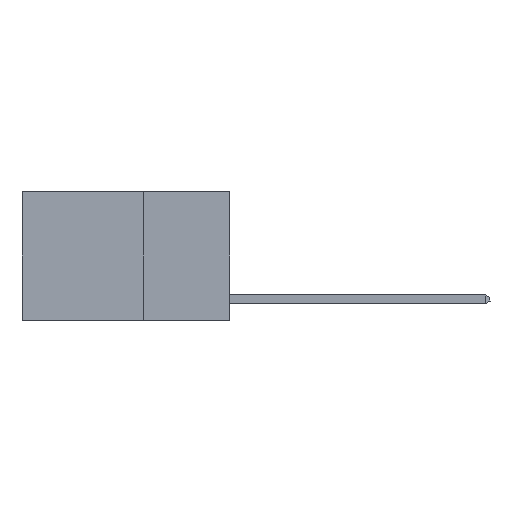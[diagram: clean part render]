
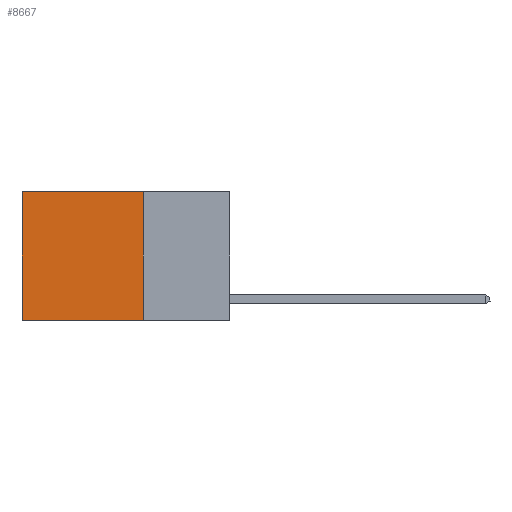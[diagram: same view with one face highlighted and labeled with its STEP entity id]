
A CAD part, left-side view. The second image highlights one B-rep face of the part: STEP entity #8667.
In plain terms, the highlighted planar face has unit normal (-1, 0, 0).
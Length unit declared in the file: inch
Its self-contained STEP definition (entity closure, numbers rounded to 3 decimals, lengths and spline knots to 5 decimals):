
#802 = VECTOR ( 'NONE', #3704, 39.37008 ) ;
#1063 = VECTOR ( 'NONE', #5669, 39.37008 ) ;
#1593 = AXIS2_PLACEMENT_3D ( 'NONE', #11629, #4308, #6087 ) ;
#1999 = VECTOR ( 'NONE', #6396, 39.37008 ) ;
#2716 = VERTEX_POINT ( 'NONE', #7676 ) ;
#2733 = CARTESIAN_POINT ( 'NONE',  ( 0.2625, 0.25, 0. ) ) ;
#3064 = EDGE_CURVE ( 'NONE', #2716, #7961, #5777, .T. ) ;
#3219 = LINE ( 'NONE', #4077, #10288 ) ;
#3458 = PLANE ( 'NONE',  #1593 ) ;
#3704 = DIRECTION ( 'NONE',  ( 0., 0., -1. ) ) ;
#4077 = CARTESIAN_POINT ( 'NONE',  ( 0.2625, 0.25, -0.37 ) ) ;
#4201 = ORIENTED_EDGE ( 'NONE', *, *, #3064, .T. ) ;
#4308 = DIRECTION ( 'NONE',  ( 1., 0., 0. ) ) ;
#4345 = LINE ( 'NONE', #11721, #1999 ) ;
#4838 = DIRECTION ( 'NONE',  ( 0., 1., 0. ) ) ;
#5084 = ORIENTED_EDGE ( 'NONE', *, *, #11746, .T. ) ;
#5361 = EDGE_LOOP ( 'NONE', ( #5084, #11357, #8856, #4201 ) ) ;
#5669 = DIRECTION ( 'NONE',  ( 0., 1., 0. ) ) ;
#5777 = LINE ( 'NONE', #11329, #1063 ) ;
#6087 = DIRECTION ( 'NONE',  ( 0., 0., -1. ) ) ;
#6196 = FACE_OUTER_BOUND ( 'NONE', #5361, .T. ) ;
#6396 = DIRECTION ( 'NONE',  ( 0., 0., -1. ) ) ;
#7013 = CARTESIAN_POINT ( 'NONE',  ( 0.2625, 0.6, -0.37 ) ) ;
#7353 = LINE ( 'NONE', #2733, #802 ) ;
#7566 = CARTESIAN_POINT ( 'NONE',  ( 0.2625, 0.6, 0. ) ) ;
#7660 = VERTEX_POINT ( 'NONE', #7013 ) ;
#7676 = CARTESIAN_POINT ( 'NONE',  ( 0.2625, 0.25, 0. ) ) ;
#7885 = VERTEX_POINT ( 'NONE', #11838 ) ;
#7961 = VERTEX_POINT ( 'NONE', #7566 ) ;
#8667 = ADVANCED_FACE ( 'NONE', ( #6196 ), #3458, .F. ) ;
#8856 = ORIENTED_EDGE ( 'NONE', *, *, #8927, .F. ) ;
#8927 = EDGE_CURVE ( 'NONE', #2716, #7885, #7353, .T. ) ;
#10288 = VECTOR ( 'NONE', #4838, 39.37008 ) ;
#11163 = EDGE_CURVE ( 'NONE', #7885, #7660, #3219, .T. ) ;
#11329 = CARTESIAN_POINT ( 'NONE',  ( 0.2625, 0.25, 0. ) ) ;
#11357 = ORIENTED_EDGE ( 'NONE', *, *, #11163, .F. ) ;
#11629 = CARTESIAN_POINT ( 'NONE',  ( 0.2625, 0.25, 0. ) ) ;
#11721 = CARTESIAN_POINT ( 'NONE',  ( 0.2625, 0.6, 0. ) ) ;
#11746 = EDGE_CURVE ( 'NONE', #7961, #7660, #4345, .T. ) ;
#11838 = CARTESIAN_POINT ( 'NONE',  ( 0.2625, 0.25, -0.37 ) ) ;
